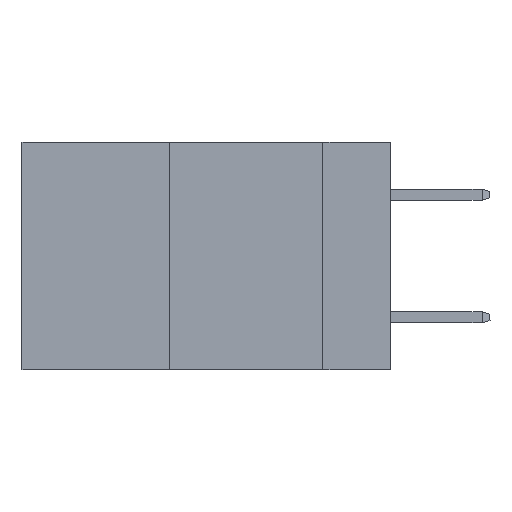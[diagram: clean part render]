
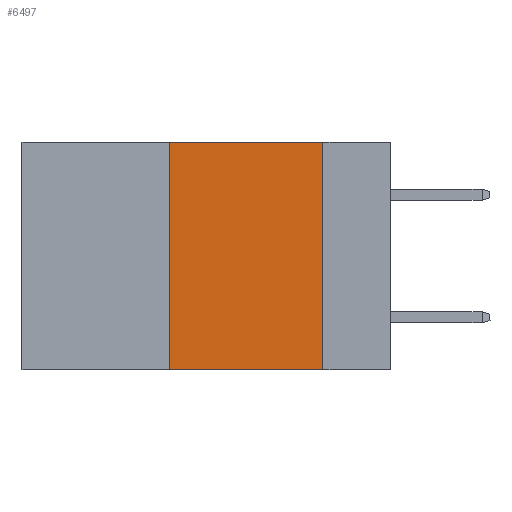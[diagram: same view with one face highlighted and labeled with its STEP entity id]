
A CAD part, left-side view. The second image highlights one B-rep face of the part: STEP entity #6497.
In plain terms, the highlighted planar face has unit normal (-1, 0, 0).
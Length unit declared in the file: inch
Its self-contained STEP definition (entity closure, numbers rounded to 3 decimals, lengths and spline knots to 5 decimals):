
#364 = EDGE_CURVE ( 'NONE', #5361, #1474, #8221, .T. ) ;
#742 = DIRECTION ( 'NONE',  ( 0., 0., -1. ) ) ;
#1099 = CARTESIAN_POINT ( 'NONE',  ( 0., 0.36, -0.37 ) ) ;
#1138 = LINE ( 'NONE', #9688, #9836 ) ;
#1290 = EDGE_CURVE ( 'NONE', #11168, #1790, #7158, .T. ) ;
#1474 = VERTEX_POINT ( 'NONE', #4427 ) ;
#1748 = CARTESIAN_POINT ( 'NONE',  ( 0., 0.6, 0. ) ) ;
#1790 = VERTEX_POINT ( 'NONE', #9576 ) ;
#1792 = DIRECTION ( 'NONE',  ( 0., -1., 0. ) ) ;
#1989 = CARTESIAN_POINT ( 'NONE',  ( 0., 0.36, 0. ) ) ;
#2693 = DIRECTION ( 'NONE',  ( 1., 0., 0. ) ) ;
#2731 = PLANE ( 'NONE',  #10525 ) ;
#3024 = ORIENTED_EDGE ( 'NONE', *, *, #364, .F. ) ;
#3074 = EDGE_CURVE ( 'NONE', #1474, #1790, #1138, .T. ) ;
#4032 = VECTOR ( 'NONE', #5880, 39.37008 ) ;
#4351 = ORIENTED_EDGE ( 'NONE', *, *, #10510, .F. ) ;
#4427 = CARTESIAN_POINT ( 'NONE',  ( 0., 0.11, 0. ) ) ;
#5230 = LINE ( 'NONE', #1989, #4032 ) ;
#5357 = CARTESIAN_POINT ( 'NONE',  ( 0., 0.36, 0. ) ) ;
#5361 = VERTEX_POINT ( 'NONE', #5357 ) ;
#5536 = VECTOR ( 'NONE', #1792, 39.37008 ) ;
#5880 = DIRECTION ( 'NONE',  ( 0., 0., 1. ) ) ;
#6497 = ADVANCED_FACE ( 'NONE', ( #10839 ), #2731, .F. ) ;
#6608 = CARTESIAN_POINT ( 'NONE',  ( 0., 0.6, 0. ) ) ;
#7053 = CARTESIAN_POINT ( 'NONE',  ( 0., 0.6, -0.37 ) ) ;
#7158 = LINE ( 'NONE', #7053, #11634 ) ;
#8221 = LINE ( 'NONE', #6608, #5536 ) ;
#8914 = DIRECTION ( 'NONE',  ( 0., 0., -1. ) ) ;
#9576 = CARTESIAN_POINT ( 'NONE',  ( 0., 0.11, -0.37 ) ) ;
#9688 = CARTESIAN_POINT ( 'NONE',  ( 0., 0.11, 0. ) ) ;
#9836 = VECTOR ( 'NONE', #8914, 39.37008 ) ;
#10510 = EDGE_CURVE ( 'NONE', #11168, #5361, #5230, .T. ) ;
#10525 = AXIS2_PLACEMENT_3D ( 'NONE', #1748, #2693, #742 ) ;
#10612 = ORIENTED_EDGE ( 'NONE', *, *, #1290, .T. ) ;
#10839 = FACE_OUTER_BOUND ( 'NONE', #12281, .T. ) ;
#11168 = VERTEX_POINT ( 'NONE', #1099 ) ;
#11634 = VECTOR ( 'NONE', #11810, 39.37008 ) ;
#11810 = DIRECTION ( 'NONE',  ( 0., -1., 0. ) ) ;
#12004 = ORIENTED_EDGE ( 'NONE', *, *, #3074, .F. ) ;
#12281 = EDGE_LOOP ( 'NONE', ( #12004, #3024, #4351, #10612 ) ) ;
